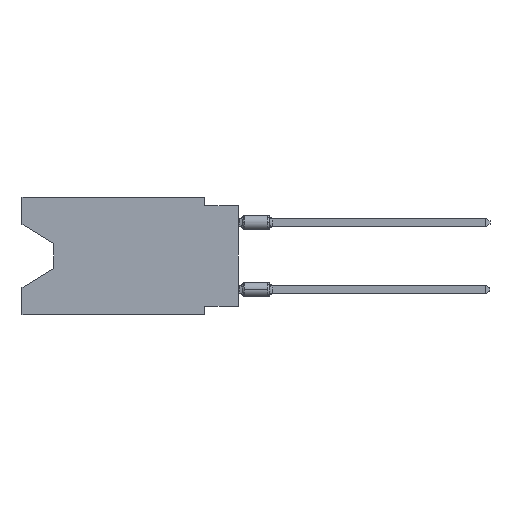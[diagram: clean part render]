
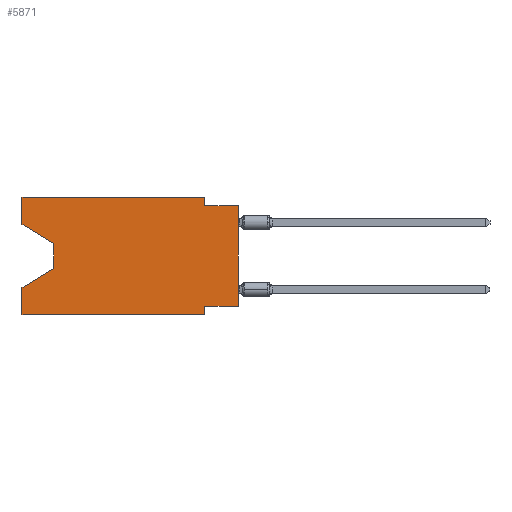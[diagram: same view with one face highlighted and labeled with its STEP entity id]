
A CAD part, left-side view. The second image highlights one B-rep face of the part: STEP entity #5871.
In plain terms, the highlighted planar face has unit normal (-1, 0, 0).
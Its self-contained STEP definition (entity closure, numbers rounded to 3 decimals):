
#475 = CARTESIAN_POINT ( 'NONE',  ( 0., 16.383, -2.038 ) ) ;
#663 = DIRECTION ( 'NONE',  ( 0., 1., 0. ) ) ;
#1333 = CARTESIAN_POINT ( 'NONE',  ( 0., 13.97, -5.385 ) ) ;
#1512 = CARTESIAN_POINT ( 'NONE',  ( 0., 13.97, -3.505 ) ) ;
#1599 = CARTESIAN_POINT ( 'NONE',  ( 0., 2.54, -8.89 ) ) ;
#1757 = VECTOR ( 'NONE', #25624, 1000. ) ;
#1760 = EDGE_CURVE ( 'NONE', #29205, #11942, #17350, .T. ) ;
#2159 = VERTEX_POINT ( 'NONE', #14862 ) ;
#2600 = EDGE_CURVE ( 'NONE', #19404, #25226, #29618, .T. ) ;
#2727 = EDGE_CURVE ( 'NONE', #10072, #6764, #19736, .T. ) ;
#3301 = CARTESIAN_POINT ( 'NONE',  ( 0., 13.97, -5.385 ) ) ;
#3398 = CARTESIAN_POINT ( 'NONE',  ( 0., 16.383, 0. ) ) ;
#3698 = VECTOR ( 'NONE', #32923, 1000. ) ;
#3726 = CARTESIAN_POINT ( 'NONE',  ( 0., 2.54, -8.255 ) ) ;
#4196 = LINE ( 'NONE', #1599, #23375 ) ;
#4231 = CARTESIAN_POINT ( 'NONE',  ( 0., 13.97, -3.505 ) ) ;
#4378 = ORIENTED_EDGE ( 'NONE', *, *, #1760, .T. ) ;
#5197 = VECTOR ( 'NONE', #30647, 1000. ) ;
#5325 = VECTOR ( 'NONE', #22328, 1000. ) ;
#5871 = ADVANCED_FACE ( 'NONE', ( #21739 ), #8599, .F. ) ;
#5912 = DIRECTION ( 'NONE',  ( 0., 0.855, -0.519 ) ) ;
#6029 = LINE ( 'NONE', #18671, #27527 ) ;
#6072 = EDGE_CURVE ( 'NONE', #10175, #18705, #14261, .T. ) ;
#6277 = ORIENTED_EDGE ( 'NONE', *, *, #24614, .T. ) ;
#6357 = EDGE_CURVE ( 'NONE', #10072, #30360, #11973, .T. ) ;
#6764 = VERTEX_POINT ( 'NONE', #25088 ) ;
#6799 = VECTOR ( 'NONE', #33736, 1000. ) ;
#8599 = PLANE ( 'NONE',  #19010 ) ;
#8625 = CARTESIAN_POINT ( 'NONE',  ( 0., 0., -8.255 ) ) ;
#8684 = DIRECTION ( 'NONE',  ( 0., 0., 1. ) ) ;
#9605 = LINE ( 'NONE', #33111, #15651 ) ;
#10072 = VERTEX_POINT ( 'NONE', #475 ) ;
#10096 = CARTESIAN_POINT ( 'NONE',  ( 0., 2.54, -0.635 ) ) ;
#10175 = VERTEX_POINT ( 'NONE', #31908 ) ;
#10886 = EDGE_CURVE ( 'NONE', #18705, #11942, #12299, .T. ) ;
#11030 = DIRECTION ( 'NONE',  ( 1., 0., 0. ) ) ;
#11123 = VECTOR ( 'NONE', #8684, 1000. ) ;
#11716 = ORIENTED_EDGE ( 'NONE', *, *, #11834, .F. ) ;
#11774 = CARTESIAN_POINT ( 'NONE',  ( 0., 16.383, -8.89 ) ) ;
#11834 = EDGE_CURVE ( 'NONE', #25601, #25226, #19914, .T. ) ;
#11942 = VERTEX_POINT ( 'NONE', #22348 ) ;
#11973 = LINE ( 'NONE', #12135, #5197 ) ;
#12135 = CARTESIAN_POINT ( 'NONE',  ( 0., 16.383, -2.038 ) ) ;
#12299 = LINE ( 'NONE', #25975, #6799 ) ;
#12943 = VECTOR ( 'NONE', #24803, 1000. ) ;
#14261 = LINE ( 'NONE', #27574, #12943 ) ;
#14601 = DIRECTION ( 'NONE',  ( 0., 0., 1. ) ) ;
#14826 = EDGE_CURVE ( 'NONE', #6764, #10175, #9605, .T. ) ;
#14862 = CARTESIAN_POINT ( 'NONE',  ( 0., 2.54, -8.89 ) ) ;
#15321 = ORIENTED_EDGE ( 'NONE', *, *, #29163, .F. ) ;
#15651 = VECTOR ( 'NONE', #30872, 1000. ) ;
#15811 = ORIENTED_EDGE ( 'NONE', *, *, #14826, .F. ) ;
#16660 = ORIENTED_EDGE ( 'NONE', *, *, #2727, .F. ) ;
#17350 = LINE ( 'NONE', #25315, #33963 ) ;
#18671 = CARTESIAN_POINT ( 'NONE',  ( 0., 0., -8.255 ) ) ;
#18705 = VERTEX_POINT ( 'NONE', #10096 ) ;
#19010 = AXIS2_PLACEMENT_3D ( 'NONE', #3398, #11030, #31954 ) ;
#19404 = VERTEX_POINT ( 'NONE', #1333 ) ;
#19723 = EDGE_CURVE ( 'NONE', #30360, #19404, #24815, .T. ) ;
#19733 = LINE ( 'NONE', #11774, #5325 ) ;
#19736 = LINE ( 'NONE', #30802, #1757 ) ;
#19914 = LINE ( 'NONE', #27722, #11123 ) ;
#20481 = EDGE_LOOP ( 'NONE', ( #30413, #20691, #24416, #11716, #6277, #27092, #15321, #4378, #29684, #27789, #15811, #16660 ) ) ;
#20691 = ORIENTED_EDGE ( 'NONE', *, *, #19723, .T. ) ;
#21391 = EDGE_CURVE ( 'NONE', #33037, #2159, #4196, .T. ) ;
#21739 = FACE_OUTER_BOUND ( 'NONE', #20481, .T. ) ;
#22328 = DIRECTION ( 'NONE',  ( 0., -1., 0. ) ) ;
#22348 = CARTESIAN_POINT ( 'NONE',  ( 0., 0., -0.635 ) ) ;
#22694 = DIRECTION ( 'NONE',  ( 0., 0., -1. ) ) ;
#23375 = VECTOR ( 'NONE', #22694, 1000. ) ;
#23396 = CARTESIAN_POINT ( 'NONE',  ( 0., 16.383, -8.89 ) ) ;
#24416 = ORIENTED_EDGE ( 'NONE', *, *, #2600, .T. ) ;
#24614 = EDGE_CURVE ( 'NONE', #25601, #2159, #19733, .T. ) ;
#24803 = DIRECTION ( 'NONE',  ( 0., 0., -1. ) ) ;
#24815 = LINE ( 'NONE', #4231, #3698 ) ;
#25088 = CARTESIAN_POINT ( 'NONE',  ( 0., 16.383, 0. ) ) ;
#25226 = VERTEX_POINT ( 'NONE', #30877 ) ;
#25315 = CARTESIAN_POINT ( 'NONE',  ( 0., 0., 0. ) ) ;
#25601 = VERTEX_POINT ( 'NONE', #23396 ) ;
#25624 = DIRECTION ( 'NONE',  ( 0., 0., 1. ) ) ;
#25975 = CARTESIAN_POINT ( 'NONE',  ( 0., 0., -0.635 ) ) ;
#27092 = ORIENTED_EDGE ( 'NONE', *, *, #21391, .F. ) ;
#27527 = VECTOR ( 'NONE', #663, 1000. ) ;
#27574 = CARTESIAN_POINT ( 'NONE',  ( 0., 2.54, 0. ) ) ;
#27722 = CARTESIAN_POINT ( 'NONE',  ( 0., 16.383, 0. ) ) ;
#27789 = ORIENTED_EDGE ( 'NONE', *, *, #6072, .F. ) ;
#29163 = EDGE_CURVE ( 'NONE', #29205, #33037, #6029, .T. ) ;
#29205 = VERTEX_POINT ( 'NONE', #8625 ) ;
#29618 = LINE ( 'NONE', #3301, #33214 ) ;
#29684 = ORIENTED_EDGE ( 'NONE', *, *, #10886, .F. ) ;
#30360 = VERTEX_POINT ( 'NONE', #1512 ) ;
#30413 = ORIENTED_EDGE ( 'NONE', *, *, #6357, .T. ) ;
#30647 = DIRECTION ( 'NONE',  ( 0., -0.855, -0.519 ) ) ;
#30802 = CARTESIAN_POINT ( 'NONE',  ( 0., 16.383, 0. ) ) ;
#30872 = DIRECTION ( 'NONE',  ( 0., -1., 0. ) ) ;
#30877 = CARTESIAN_POINT ( 'NONE',  ( 0., 16.383, -6.852 ) ) ;
#31908 = CARTESIAN_POINT ( 'NONE',  ( 0., 2.54, 0. ) ) ;
#31954 = DIRECTION ( 'NONE',  ( 0., 0., -1. ) ) ;
#32923 = DIRECTION ( 'NONE',  ( 0., 0., -1. ) ) ;
#33037 = VERTEX_POINT ( 'NONE', #3726 ) ;
#33111 = CARTESIAN_POINT ( 'NONE',  ( 0., 16.383, 0. ) ) ;
#33214 = VECTOR ( 'NONE', #5912, 1000. ) ;
#33736 = DIRECTION ( 'NONE',  ( 0., -1., 0. ) ) ;
#33963 = VECTOR ( 'NONE', #14601, 1000. ) ;
